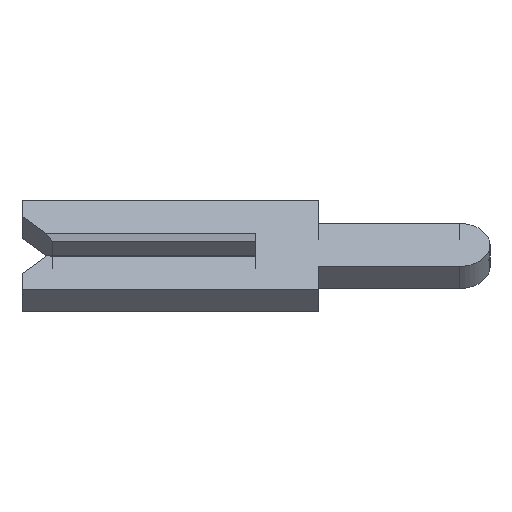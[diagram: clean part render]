
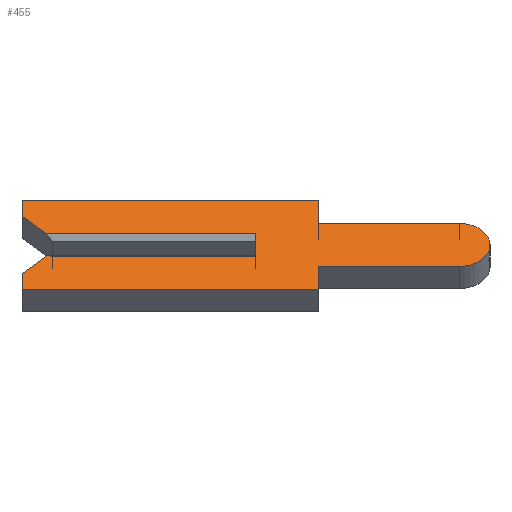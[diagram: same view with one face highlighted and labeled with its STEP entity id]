
A CAD part, left-side view. The second image highlights one B-rep face of the part: STEP entity #455.
In plain terms, the highlighted face is planar.
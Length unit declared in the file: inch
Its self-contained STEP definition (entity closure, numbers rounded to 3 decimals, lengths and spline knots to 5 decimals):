
#42 = CARTESIAN_POINT ( 'NONE',  ( -0.01, 0.1305, -0.0065 ) ) ;
#52 = DIRECTION ( 'NONE',  ( 0., 0., -1. ) ) ;
#78 = VECTOR ( 'NONE', #2196, 39.37008 ) ;
#92 = LINE ( 'NONE', #1183, #1586 ) ;
#114 = EDGE_CURVE ( 'NONE', #2244, #761, #1120, .T. ) ;
#201 = DIRECTION ( 'NONE',  ( 0., -1., 0. ) ) ;
#235 = ORIENTED_EDGE ( 'NONE', *, *, #2351, .F. ) ;
#238 = EDGE_CURVE ( 'NONE', #1993, #1865, #1743, .T. ) ;
#240 = CARTESIAN_POINT ( 'NONE',  ( -0.01, 0., 0.0065 ) ) ;
#283 = LINE ( 'NONE', #529, #1133 ) ;
#293 = ORIENTED_EDGE ( 'NONE', *, *, #370, .F. ) ;
#370 = EDGE_CURVE ( 'NONE', #1718, #1919, #2107, .T. ) ;
#379 = CIRCLE ( 'NONE', #1954, 0.0195 ) ;
#392 = CARTESIAN_POINT ( 'NONE',  ( -0.01, 0.15, 0.04 ) ) ;
#401 = ORIENTED_EDGE ( 'NONE', *, *, #1212, .F. ) ;
#417 = CARTESIAN_POINT ( 'NONE',  ( -0.01, -0.04, 0.0195 ) ) ;
#436 = EDGE_CURVE ( 'NONE', #1313, #1718, #788, .T. ) ;
#455 = ADVANCED_FACE ( 'NONE', ( #1801 ), #2053, .F. ) ;
#465 = VECTOR ( 'NONE', #1395, 39.37008 ) ;
#529 = CARTESIAN_POINT ( 'NONE',  ( -0.01, 0.1305, 0.0065 ) ) ;
#538 = CARTESIAN_POINT ( 'NONE',  ( -0.01, 0.134, 0.01 ) ) ;
#544 = CARTESIAN_POINT ( 'NONE',  ( -0.01, -0.1305, 0.0195 ) ) ;
#561 = CARTESIAN_POINT ( 'NONE',  ( -0.01, -0.1305, -0.0195 ) ) ;
#622 = LINE ( 'NONE', #2449, #1618 ) ;
#645 = CARTESIAN_POINT ( 'NONE',  ( -0.01, 0.15, 0.026 ) ) ;
#653 = LINE ( 'NONE', #1518, #1161 ) ;
#669 = ORIENTED_EDGE ( 'NONE', *, *, #1086, .F. ) ;
#675 = ORIENTED_EDGE ( 'NONE', *, *, #875, .F. ) ;
#706 = VECTOR ( 'NONE', #1020, 39.37008 ) ;
#731 = ORIENTED_EDGE ( 'NONE', *, *, #1655, .F. ) ;
#737 = ORIENTED_EDGE ( 'NONE', *, *, #436, .F. ) ;
#761 = VERTEX_POINT ( 'NONE', #1447 ) ;
#788 = LINE ( 'NONE', #1823, #1603 ) ;
#792 = CARTESIAN_POINT ( 'NONE',  ( -0.01, -0.04, -0.0195 ) ) ;
#812 = VERTEX_POINT ( 'NONE', #1055 ) ;
#814 = CARTESIAN_POINT ( 'NONE',  ( -0.01, 0.15, 0.01 ) ) ;
#822 = DIRECTION ( 'NONE',  ( 1., 0., 0. ) ) ;
#875 = EDGE_CURVE ( 'NONE', #2426, #2301, #622, .T. ) ;
#911 = CARTESIAN_POINT ( 'NONE',  ( -0.01, 0.15, -0.04 ) ) ;
#926 = DIRECTION ( 'NONE',  ( 0., 0., -1. ) ) ;
#941 = ORIENTED_EDGE ( 'NONE', *, *, #114, .F. ) ;
#947 = VERTEX_POINT ( 'NONE', #538 ) ;
#959 = EDGE_CURVE ( 'NONE', #1609, #1926, #1424, .T. ) ;
#977 = EDGE_CURVE ( 'NONE', #1919, #1609, #1688, .T. ) ;
#1001 = DIRECTION ( 'NONE',  ( 0., 0., -1. ) ) ;
#1020 = DIRECTION ( 'NONE',  ( 0., 0., 1. ) ) ;
#1029 = VECTOR ( 'NONE', #2015, 39.37008 ) ;
#1055 = CARTESIAN_POINT ( 'NONE',  ( -0.01, 0.134, -0.01 ) ) ;
#1069 = ORIENTED_EDGE ( 'NONE', *, *, #1796, .T. ) ;
#1086 = EDGE_CURVE ( 'NONE', #947, #1993, #283, .T. ) ;
#1106 = LINE ( 'NONE', #814, #1492 ) ;
#1120 = LINE ( 'NONE', #240, #706 ) ;
#1133 = VECTOR ( 'NONE', #2486, 39.37008 ) ;
#1161 = VECTOR ( 'NONE', #2116, 39.37008 ) ;
#1170 = CARTESIAN_POINT ( 'NONE',  ( -0.01, 0.15, 0.026 ) ) ;
#1183 = CARTESIAN_POINT ( 'NONE',  ( -0.01, -0.04, 0.0195 ) ) ;
#1212 = EDGE_CURVE ( 'NONE', #1865, #2426, #653, .T. ) ;
#1214 = ORIENTED_EDGE ( 'NONE', *, *, #238, .F. ) ;
#1236 = DIRECTION ( 'NONE',  ( 0., 1., 0. ) ) ;
#1306 = ORIENTED_EDGE ( 'NONE', *, *, #977, .F. ) ;
#1313 = VERTEX_POINT ( 'NONE', #561 ) ;
#1323 = CARTESIAN_POINT ( 'NONE',  ( -0.01, 0.15, -0.04 ) ) ;
#1332 = VECTOR ( 'NONE', #52, 39.37008 ) ;
#1395 = DIRECTION ( 'NONE',  ( 0., -0.707, 0.707 ) ) ;
#1420 = VERTEX_POINT ( 'NONE', #544 ) ;
#1424 = LINE ( 'NONE', #1893, #2056 ) ;
#1440 = CARTESIAN_POINT ( 'NONE',  ( -0.01, -0.04, -0.04 ) ) ;
#1447 = CARTESIAN_POINT ( 'NONE',  ( -0.01, 0., 0.01 ) ) ;
#1483 = DIRECTION ( 'NONE',  ( 0., 1., 0. ) ) ;
#1492 = VECTOR ( 'NONE', #2161, 39.37008 ) ;
#1518 = CARTESIAN_POINT ( 'NONE',  ( -0.01, 0.15, 0.04 ) ) ;
#1586 = VECTOR ( 'NONE', #201, 39.37008 ) ;
#1603 = VECTOR ( 'NONE', #1236, 39.37008 ) ;
#1609 = VERTEX_POINT ( 'NONE', #1323 ) ;
#1615 = CARTESIAN_POINT ( 'NONE',  ( -0.01, -0.1305, 0. ) ) ;
#1618 = VECTOR ( 'NONE', #926, 39.37008 ) ;
#1650 = LINE ( 'NONE', #2194, #1029 ) ;
#1655 = EDGE_CURVE ( 'NONE', #2301, #1420, #92, .T. ) ;
#1688 = LINE ( 'NONE', #911, #2092 ) ;
#1718 = VERTEX_POINT ( 'NONE', #792 ) ;
#1736 = ORIENTED_EDGE ( 'NONE', *, *, #959, .F. ) ;
#1743 = LINE ( 'NONE', #645, #78 ) ;
#1759 = CARTESIAN_POINT ( 'NONE',  ( -0.01, -0.04, -0.04 ) ) ;
#1778 = ORIENTED_EDGE ( 'NONE', *, *, #2273, .F. ) ;
#1796 = EDGE_CURVE ( 'NONE', #947, #761, #1106, .T. ) ;
#1801 = FACE_OUTER_BOUND ( 'NONE', #1871, .T. ) ;
#1815 = CARTESIAN_POINT ( 'NONE',  ( -0.01, -0.1305, 0. ) ) ;
#1823 = CARTESIAN_POINT ( 'NONE',  ( -0.01, -0.04, -0.0195 ) ) ;
#1865 = VERTEX_POINT ( 'NONE', #392 ) ;
#1871 = EDGE_LOOP ( 'NONE', ( #1069, #941, #235, #2459, #1736, #1306, #293, #737, #1778, #731, #675, #401, #1214, #669 ) ) ;
#1872 = LINE ( 'NONE', #42, #465 ) ;
#1893 = CARTESIAN_POINT ( 'NONE',  ( -0.01, 0.15, -0.026 ) ) ;
#1919 = VERTEX_POINT ( 'NONE', #1759 ) ;
#1926 = VERTEX_POINT ( 'NONE', #2352 ) ;
#1954 = AXIS2_PLACEMENT_3D ( 'NONE', #1815, #822, #1001 ) ;
#1993 = VERTEX_POINT ( 'NONE', #1170 ) ;
#2015 = DIRECTION ( 'NONE',  ( 0., -1., 0. ) ) ;
#2017 = DIRECTION ( 'NONE',  ( 0., 0., -1. ) ) ;
#2020 = CARTESIAN_POINT ( 'NONE',  ( -0.01, 0., -0.01 ) ) ;
#2053 = PLANE ( 'NONE',  #2259 ) ;
#2056 = VECTOR ( 'NONE', #2073, 39.37008 ) ;
#2073 = DIRECTION ( 'NONE',  ( 0., 0., 1. ) ) ;
#2092 = VECTOR ( 'NONE', #1483, 39.37008 ) ;
#2107 = LINE ( 'NONE', #1440, #1332 ) ;
#2116 = DIRECTION ( 'NONE',  ( 0., -1., 0. ) ) ;
#2161 = DIRECTION ( 'NONE',  ( 0., -1., 0. ) ) ;
#2194 = CARTESIAN_POINT ( 'NONE',  ( -0.01, -0.1305, -0.01 ) ) ;
#2196 = DIRECTION ( 'NONE',  ( 0., 0., 1. ) ) ;
#2244 = VERTEX_POINT ( 'NONE', #2020 ) ;
#2252 = DIRECTION ( 'NONE',  ( 1., 0., 0. ) ) ;
#2259 = AXIS2_PLACEMENT_3D ( 'NONE', #1615, #2252, #2017 ) ;
#2273 = EDGE_CURVE ( 'NONE', #1420, #1313, #379, .T. ) ;
#2301 = VERTEX_POINT ( 'NONE', #417 ) ;
#2351 = EDGE_CURVE ( 'NONE', #812, #2244, #1650, .T. ) ;
#2352 = CARTESIAN_POINT ( 'NONE',  ( -0.01, 0.15, -0.026 ) ) ;
#2384 = EDGE_CURVE ( 'NONE', #1926, #812, #1872, .T. ) ;
#2409 = CARTESIAN_POINT ( 'NONE',  ( -0.01, -0.04, 0.04 ) ) ;
#2426 = VERTEX_POINT ( 'NONE', #2409 ) ;
#2449 = CARTESIAN_POINT ( 'NONE',  ( -0.01, -0.04, 0.04 ) ) ;
#2459 = ORIENTED_EDGE ( 'NONE', *, *, #2384, .F. ) ;
#2486 = DIRECTION ( 'NONE',  ( 0., 0.707, 0.707 ) ) ;
